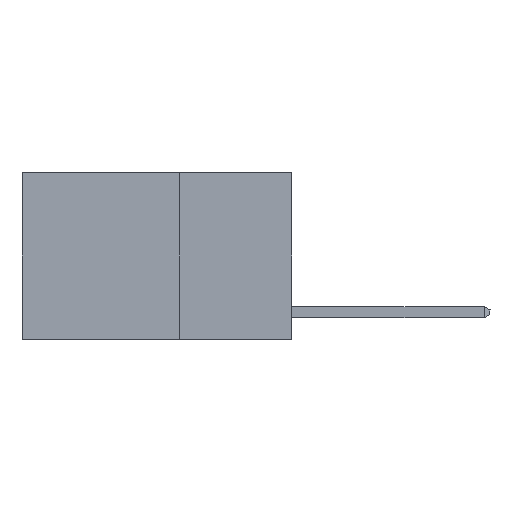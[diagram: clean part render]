
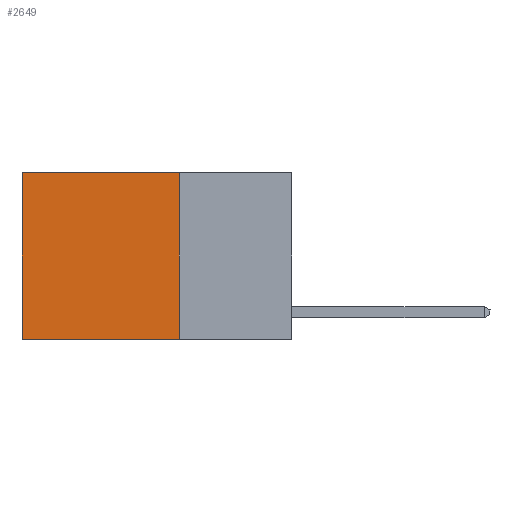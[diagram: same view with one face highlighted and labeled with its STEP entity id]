
A CAD part, left-side view. The second image highlights one B-rep face of the part: STEP entity #2649.
In plain terms, the highlighted planar face has unit normal (-1, 0, 0).
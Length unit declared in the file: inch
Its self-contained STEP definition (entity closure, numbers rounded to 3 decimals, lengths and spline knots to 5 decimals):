
#564 = CARTESIAN_POINT ( 'NONE',  ( 0.2625, 0.25, -0.37 ) ) ;
#565 = CARTESIAN_POINT ( 'NONE',  ( 0.2625, 0.25, 0. ) ) ;
#1221 = VECTOR ( 'NONE', #12252, 39.37008 ) ;
#1396 = DIRECTION ( 'NONE',  ( 1., 0., 0. ) ) ;
#1461 = EDGE_CURVE ( 'NONE', #2695, #13580, #11648, .T. ) ;
#1768 = DIRECTION ( 'NONE',  ( 0., 1., 0. ) ) ;
#2432 = EDGE_LOOP ( 'NONE', ( #5235, #6119, #7899, #14448 ) ) ;
#2649 = ADVANCED_FACE ( 'NONE', ( #12661 ), #2950, .F. ) ;
#2695 = VERTEX_POINT ( 'NONE', #564 ) ;
#2950 = PLANE ( 'NONE',  #8766 ) ;
#4011 = VECTOR ( 'NONE', #1768, 39.37008 ) ;
#4267 = LINE ( 'NONE', #565, #1221 ) ;
#4385 = EDGE_CURVE ( 'NONE', #10431, #6183, #12966, .T. ) ;
#4665 = CARTESIAN_POINT ( 'NONE',  ( 0.2625, 0.6, -0.37 ) ) ;
#5197 = LINE ( 'NONE', #8172, #8031 ) ;
#5235 = ORIENTED_EDGE ( 'NONE', *, *, #8980, .T. ) ;
#6119 = ORIENTED_EDGE ( 'NONE', *, *, #1461, .F. ) ;
#6183 = VERTEX_POINT ( 'NONE', #11009 ) ;
#6907 = DIRECTION ( 'NONE',  ( 0., 1., 0. ) ) ;
#7791 = DIRECTION ( 'NONE',  ( 0., 0., -1. ) ) ;
#7899 = ORIENTED_EDGE ( 'NONE', *, *, #10172, .F. ) ;
#7901 = CARTESIAN_POINT ( 'NONE',  ( 0.2625, 0.25, 0. ) ) ;
#8031 = VECTOR ( 'NONE', #13842, 39.37008 ) ;
#8172 = CARTESIAN_POINT ( 'NONE',  ( 0.2625, 0.6, 0. ) ) ;
#8766 = AXIS2_PLACEMENT_3D ( 'NONE', #7901, #1396, #7791 ) ;
#8980 = EDGE_CURVE ( 'NONE', #6183, #13580, #5197, .T. ) ;
#10011 = CARTESIAN_POINT ( 'NONE',  ( 0.2625, 0.25, 0. ) ) ;
#10172 = EDGE_CURVE ( 'NONE', #10431, #2695, #4267, .T. ) ;
#10431 = VERTEX_POINT ( 'NONE', #13827 ) ;
#11009 = CARTESIAN_POINT ( 'NONE',  ( 0.2625, 0.6, 0. ) ) ;
#11648 = LINE ( 'NONE', #14255, #14556 ) ;
#12252 = DIRECTION ( 'NONE',  ( 0., 0., -1. ) ) ;
#12661 = FACE_OUTER_BOUND ( 'NONE', #2432, .T. ) ;
#12966 = LINE ( 'NONE', #10011, #4011 ) ;
#13580 = VERTEX_POINT ( 'NONE', #4665 ) ;
#13827 = CARTESIAN_POINT ( 'NONE',  ( 0.2625, 0.25, 0. ) ) ;
#13842 = DIRECTION ( 'NONE',  ( 0., 0., -1. ) ) ;
#14255 = CARTESIAN_POINT ( 'NONE',  ( 0.2625, 0.25, -0.37 ) ) ;
#14448 = ORIENTED_EDGE ( 'NONE', *, *, #4385, .T. ) ;
#14556 = VECTOR ( 'NONE', #6907, 39.37008 ) ;
